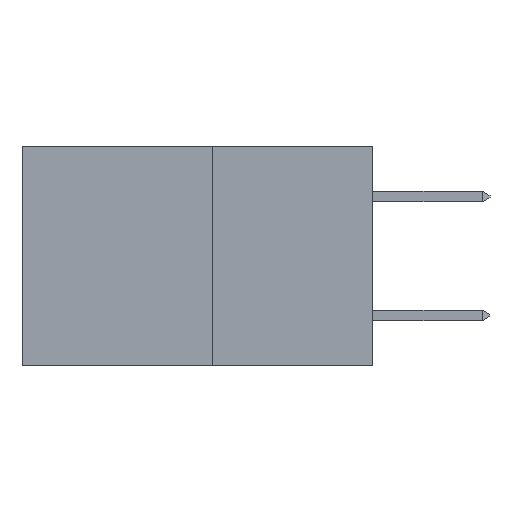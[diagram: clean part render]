
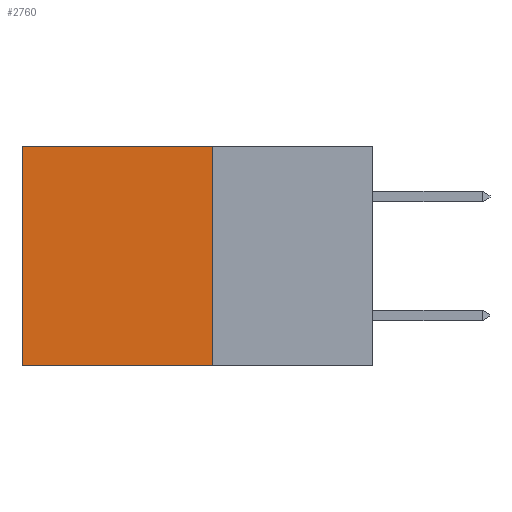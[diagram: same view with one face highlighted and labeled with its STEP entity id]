
A CAD part, left-side view. The second image highlights one B-rep face of the part: STEP entity #2760.
In plain terms, the highlighted planar face has unit normal (-1, 0, 0).
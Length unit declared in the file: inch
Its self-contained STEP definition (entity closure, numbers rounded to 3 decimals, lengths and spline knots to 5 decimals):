
#34 = FACE_OUTER_BOUND ( 'NONE', #471, .T. ) ;
#142 = VECTOR ( 'NONE', #5507, 39.37008 ) ;
#471 = EDGE_LOOP ( 'NONE', ( #6451, #3357, #2636, #5231 ) ) ;
#550 = VERTEX_POINT ( 'NONE', #6347 ) ;
#611 = VERTEX_POINT ( 'NONE', #7338 ) ;
#770 = LINE ( 'NONE', #4024, #6999 ) ;
#795 = EDGE_CURVE ( 'NONE', #1671, #550, #770, .T. ) ;
#894 = CARTESIAN_POINT ( 'NONE',  ( 0.277, 0.59, -0.37 ) ) ;
#1156 = DIRECTION ( 'NONE',  ( 0., 0., -1. ) ) ;
#1325 = AXIS2_PLACEMENT_3D ( 'NONE', #6964, #6872, #1156 ) ;
#1671 = VERTEX_POINT ( 'NONE', #3042 ) ;
#1908 = PLANE ( 'NONE',  #1325 ) ;
#2636 = ORIENTED_EDGE ( 'NONE', *, *, #4208, .F. ) ;
#2752 = DIRECTION ( 'NONE',  ( 0., 1., 0. ) ) ;
#2760 = ADVANCED_FACE ( 'NONE', ( #34 ), #1908, .F. ) ;
#2773 = DIRECTION ( 'NONE',  ( 0., 0., -1. ) ) ;
#3042 = CARTESIAN_POINT ( 'NONE',  ( 0.277, 0.27, 0. ) ) ;
#3157 = EDGE_CURVE ( 'NONE', #611, #3873, #4223, .T. ) ;
#3357 = ORIENTED_EDGE ( 'NONE', *, *, #3157, .F. ) ;
#3873 = VERTEX_POINT ( 'NONE', #894 ) ;
#4024 = CARTESIAN_POINT ( 'NONE',  ( 0.277, 0.27, 0. ) ) ;
#4208 = EDGE_CURVE ( 'NONE', #1671, #611, #7424, .T. ) ;
#4223 = LINE ( 'NONE', #5468, #142 ) ;
#4485 = CARTESIAN_POINT ( 'NONE',  ( 0.277, 0.27, -0.37 ) ) ;
#5104 = EDGE_CURVE ( 'NONE', #550, #3873, #7161, .T. ) ;
#5231 = ORIENTED_EDGE ( 'NONE', *, *, #795, .T. ) ;
#5468 = CARTESIAN_POINT ( 'NONE',  ( 0.277, 0.27, -0.37 ) ) ;
#5507 = DIRECTION ( 'NONE',  ( 0., 1., 0. ) ) ;
#6046 = VECTOR ( 'NONE', #7374, 39.37008 ) ;
#6347 = CARTESIAN_POINT ( 'NONE',  ( 0.277, 0.59, 0. ) ) ;
#6451 = ORIENTED_EDGE ( 'NONE', *, *, #5104, .T. ) ;
#6648 = VECTOR ( 'NONE', #2773, 39.37008 ) ;
#6872 = DIRECTION ( 'NONE',  ( 1., 0., 0. ) ) ;
#6889 = CARTESIAN_POINT ( 'NONE',  ( 0.277, 0.59, -0.37 ) ) ;
#6964 = CARTESIAN_POINT ( 'NONE',  ( 0.277, 0.27, -0.37 ) ) ;
#6999 = VECTOR ( 'NONE', #2752, 39.37008 ) ;
#7161 = LINE ( 'NONE', #6889, #6648 ) ;
#7338 = CARTESIAN_POINT ( 'NONE',  ( 0.277, 0.27, -0.37 ) ) ;
#7374 = DIRECTION ( 'NONE',  ( 0., 0., -1. ) ) ;
#7424 = LINE ( 'NONE', #4485, #6046 ) ;
